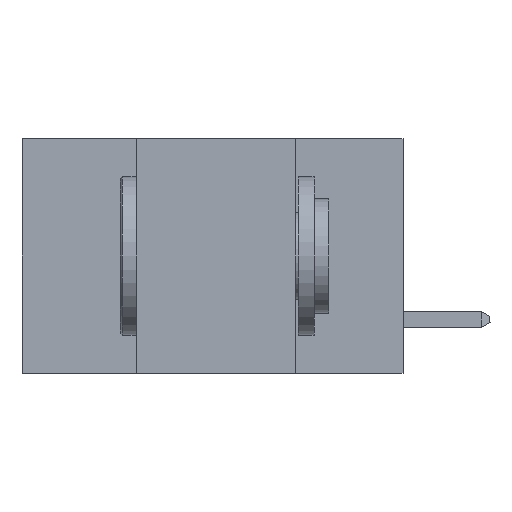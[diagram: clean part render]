
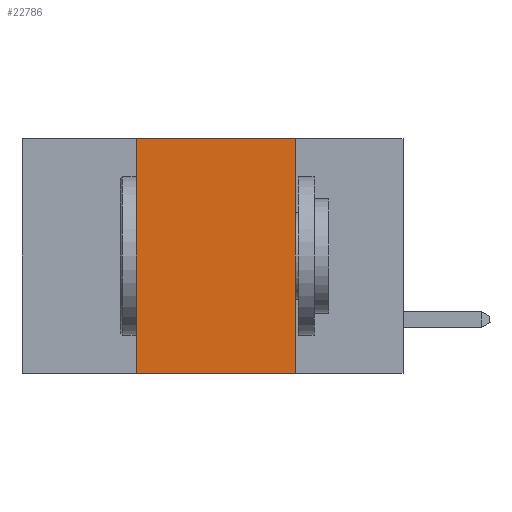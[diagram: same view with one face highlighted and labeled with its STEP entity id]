
A CAD part, left-side view. The second image highlights one B-rep face of the part: STEP entity #22786.
In plain terms, the highlighted planar face has unit normal (-1, 0, 0).
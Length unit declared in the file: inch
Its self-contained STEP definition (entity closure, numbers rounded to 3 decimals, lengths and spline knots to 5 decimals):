
#1705 = CARTESIAN_POINT ( 'NONE',  ( 0., 0.42, 0. ) ) ;
#2366 = EDGE_CURVE ( 'NONE', #2621, #9465, #13724, .T. ) ;
#2621 = VERTEX_POINT ( 'NONE', #5892 ) ;
#3217 = CARTESIAN_POINT ( 'NONE',  ( 0., 0.6, 0. ) ) ;
#4018 = CARTESIAN_POINT ( 'NONE',  ( 0., 0.17, 0. ) ) ;
#5811 = EDGE_CURVE ( 'NONE', #2621, #13142, #20054, .T. ) ;
#5892 = CARTESIAN_POINT ( 'NONE',  ( 0., 0.42, -0.37 ) ) ;
#7373 = EDGE_LOOP ( 'NONE', ( #34931, #12054, #13259, #39008 ) ) ;
#9465 = VERTEX_POINT ( 'NONE', #37644 ) ;
#9546 = LINE ( 'NONE', #18419, #15798 ) ;
#12054 = ORIENTED_EDGE ( 'NONE', *, *, #21899, .F. ) ;
#13142 = VERTEX_POINT ( 'NONE', #16844 ) ;
#13259 = ORIENTED_EDGE ( 'NONE', *, *, #2366, .F. ) ;
#13724 = LINE ( 'NONE', #1705, #20930 ) ;
#14815 = CARTESIAN_POINT ( 'NONE',  ( 0., 0.6, -0.37 ) ) ;
#15798 = VECTOR ( 'NONE', #21495, 39.37008 ) ;
#16844 = CARTESIAN_POINT ( 'NONE',  ( 0., 0.17, -0.37 ) ) ;
#17477 = DIRECTION ( 'NONE',  ( 0., 0., -1. ) ) ;
#17914 = DIRECTION ( 'NONE',  ( 0., -1., 0. ) ) ;
#18317 = VERTEX_POINT ( 'NONE', #4018 ) ;
#18419 = CARTESIAN_POINT ( 'NONE',  ( 0., 0.17, 0. ) ) ;
#20054 = LINE ( 'NONE', #14815, #27242 ) ;
#20930 = VECTOR ( 'NONE', #35435, 39.37008 ) ;
#21495 = DIRECTION ( 'NONE',  ( 0., 0., -1. ) ) ;
#21899 = EDGE_CURVE ( 'NONE', #9465, #18317, #23992, .T. ) ;
#22786 = ADVANCED_FACE ( 'NONE', ( #37833 ), #29637, .F. ) ;
#23034 = VECTOR ( 'NONE', #36939, 39.37008 ) ;
#23992 = LINE ( 'NONE', #3217, #23034 ) ;
#27242 = VECTOR ( 'NONE', #17914, 39.37008 ) ;
#29637 = PLANE ( 'NONE',  #36838 ) ;
#32725 = CARTESIAN_POINT ( 'NONE',  ( 0., 0.6, 0. ) ) ;
#34931 = ORIENTED_EDGE ( 'NONE', *, *, #38821, .F. ) ;
#35435 = DIRECTION ( 'NONE',  ( 0., 0., 1. ) ) ;
#35802 = DIRECTION ( 'NONE',  ( 1., 0., 0. ) ) ;
#36838 = AXIS2_PLACEMENT_3D ( 'NONE', #32725, #35802, #17477 ) ;
#36939 = DIRECTION ( 'NONE',  ( 0., -1., 0. ) ) ;
#37644 = CARTESIAN_POINT ( 'NONE',  ( 0., 0.42, 0. ) ) ;
#37833 = FACE_OUTER_BOUND ( 'NONE', #7373, .T. ) ;
#38821 = EDGE_CURVE ( 'NONE', #18317, #13142, #9546, .T. ) ;
#39008 = ORIENTED_EDGE ( 'NONE', *, *, #5811, .T. ) ;
